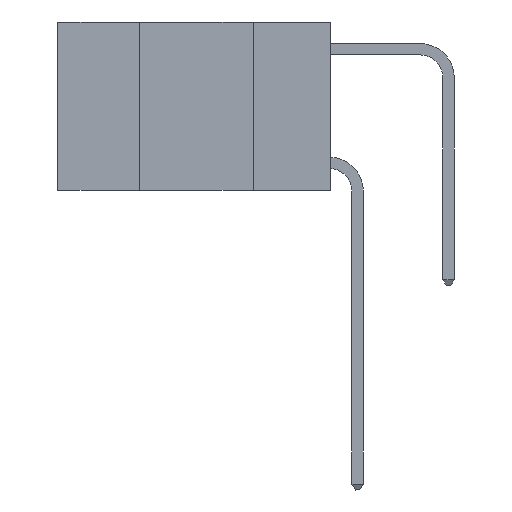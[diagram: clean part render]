
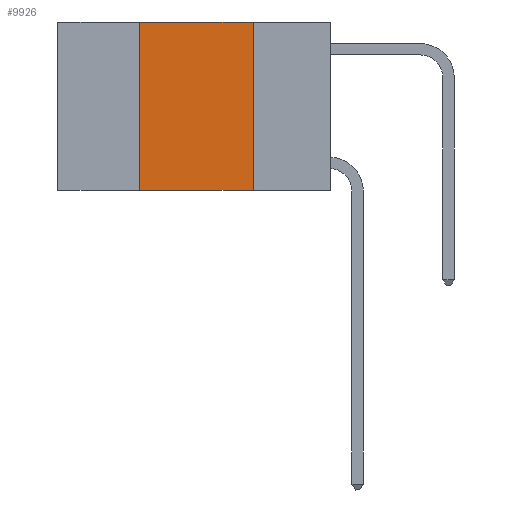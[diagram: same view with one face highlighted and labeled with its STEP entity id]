
A CAD part, left-side view. The second image highlights one B-rep face of the part: STEP entity #9926.
In plain terms, the highlighted planar face has unit normal (-1, 0, 0).
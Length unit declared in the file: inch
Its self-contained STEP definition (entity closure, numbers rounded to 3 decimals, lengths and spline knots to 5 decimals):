
#16 = EDGE_CURVE ( 'NONE', #12716, #10592, #14747, .T. ) ;
#2152 = CARTESIAN_POINT ( 'NONE',  ( 0., 0.42, -0.37 ) ) ;
#3104 = LINE ( 'NONE', #20631, #19932 ) ;
#3322 = CARTESIAN_POINT ( 'NONE',  ( 0., 0.17, 0. ) ) ;
#3705 = DIRECTION ( 'NONE',  ( 0., 0., -1. ) ) ;
#4291 = CARTESIAN_POINT ( 'NONE',  ( 0., 0.6, 0. ) ) ;
#4612 = EDGE_CURVE ( 'NONE', #15812, #9760, #7297, .T. ) ;
#5628 = VECTOR ( 'NONE', #6876, 39.37008 ) ;
#5677 = ORIENTED_EDGE ( 'NONE', *, *, #7085, .F. ) ;
#6876 = DIRECTION ( 'NONE',  ( 0., 0., -1. ) ) ;
#6978 = VECTOR ( 'NONE', #16193, 39.37008 ) ;
#7085 = EDGE_CURVE ( 'NONE', #10592, #9760, #8778, .T. ) ;
#7297 = LINE ( 'NONE', #10817, #6978 ) ;
#7749 = ORIENTED_EDGE ( 'NONE', *, *, #15130, .F. ) ;
#8110 = ORIENTED_EDGE ( 'NONE', *, *, #16, .F. ) ;
#8605 = AXIS2_PLACEMENT_3D ( 'NONE', #4291, #21196, #3705 ) ;
#8778 = LINE ( 'NONE', #3322, #5628 ) ;
#9760 = VERTEX_POINT ( 'NONE', #11035 ) ;
#9926 = ADVANCED_FACE ( 'NONE', ( #19765 ), #19870, .F. ) ;
#10592 = VERTEX_POINT ( 'NONE', #16527 ) ;
#10817 = CARTESIAN_POINT ( 'NONE',  ( 0., 0.6, -0.37 ) ) ;
#11035 = CARTESIAN_POINT ( 'NONE',  ( 0., 0.17, -0.37 ) ) ;
#11279 = DIRECTION ( 'NONE',  ( 0., -1., 0. ) ) ;
#11431 = ORIENTED_EDGE ( 'NONE', *, *, #4612, .T. ) ;
#12716 = VERTEX_POINT ( 'NONE', #20410 ) ;
#14747 = LINE ( 'NONE', #21654, #17923 ) ;
#15130 = EDGE_CURVE ( 'NONE', #15812, #12716, #3104, .T. ) ;
#15812 = VERTEX_POINT ( 'NONE', #2152 ) ;
#16193 = DIRECTION ( 'NONE',  ( 0., -1., 0. ) ) ;
#16527 = CARTESIAN_POINT ( 'NONE',  ( 0., 0.17, 0. ) ) ;
#17923 = VECTOR ( 'NONE', #11279, 39.37008 ) ;
#18923 = DIRECTION ( 'NONE',  ( 0., 0., 1. ) ) ;
#19765 = FACE_OUTER_BOUND ( 'NONE', #21120, .T. ) ;
#19870 = PLANE ( 'NONE',  #8605 ) ;
#19932 = VECTOR ( 'NONE', #18923, 39.37008 ) ;
#20410 = CARTESIAN_POINT ( 'NONE',  ( 0., 0.42, 0. ) ) ;
#20631 = CARTESIAN_POINT ( 'NONE',  ( 0., 0.42, 0. ) ) ;
#21120 = EDGE_LOOP ( 'NONE', ( #5677, #8110, #7749, #11431 ) ) ;
#21196 = DIRECTION ( 'NONE',  ( 1., 0., 0. ) ) ;
#21654 = CARTESIAN_POINT ( 'NONE',  ( 0., 0.6, 0. ) ) ;
